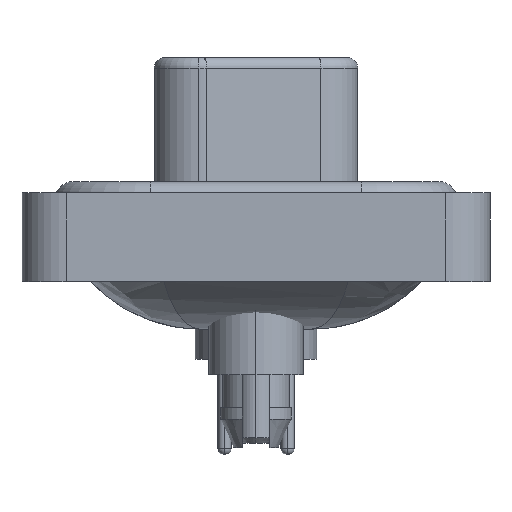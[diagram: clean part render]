
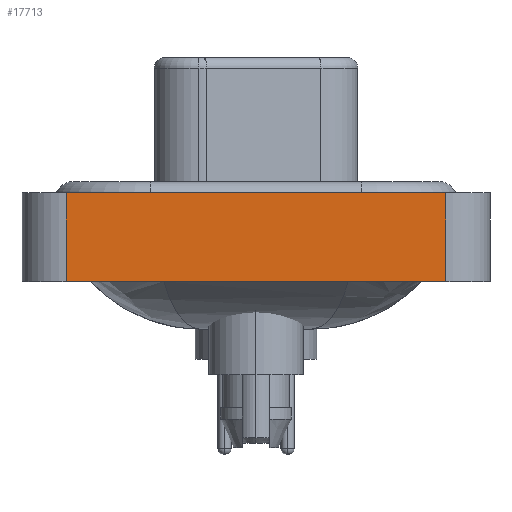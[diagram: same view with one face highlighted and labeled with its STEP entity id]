
A CAD part, left-side view. The second image highlights one B-rep face of the part: STEP entity #17713.
In plain terms, the highlighted planar face has unit normal (-1, 0, 0).
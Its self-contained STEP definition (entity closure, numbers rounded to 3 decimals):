
#1479 = VECTOR ( 'NONE', #15555, 1000. ) ;
#1630 = LINE ( 'NONE', #17493, #13610 ) ;
#1806 = PLANE ( 'NONE',  #7058 ) ;
#2822 = EDGE_LOOP ( 'NONE', ( #3918, #4203, #17969, #15794 ) ) ;
#3918 = ORIENTED_EDGE ( 'NONE', *, *, #9769, .T. ) ;
#4203 = ORIENTED_EDGE ( 'NONE', *, *, #18684, .F. ) ;
#5059 = VERTEX_POINT ( 'NONE', #7297 ) ;
#5425 = CARTESIAN_POINT ( 'NONE',  ( -7.35, -8.55, -3.6 ) ) ;
#6991 = CARTESIAN_POINT ( 'NONE',  ( -7.35, -8.55, -3.6 ) ) ;
#7058 = AXIS2_PLACEMENT_3D ( 'NONE', #6991, #20671, #15852 ) ;
#7297 = CARTESIAN_POINT ( 'NONE',  ( -7.35, -8.55, 0.4 ) ) ;
#8359 = CARTESIAN_POINT ( 'NONE',  ( -7.35, -8.55, -3.6 ) ) ;
#8612 = CARTESIAN_POINT ( 'NONE',  ( -7.35, 8.55, -3.6 ) ) ;
#9769 = EDGE_CURVE ( 'NONE', #21644, #5059, #1630, .T. ) ;
#9813 = EDGE_CURVE ( 'NONE', #21570, #21644, #10720, .T. ) ;
#10720 = LINE ( 'NONE', #5425, #1479 ) ;
#10827 = CARTESIAN_POINT ( 'NONE',  ( -7.35, -8.55, 0.4 ) ) ;
#12209 = CARTESIAN_POINT ( 'NONE',  ( -7.35, 8.55, 0.4 ) ) ;
#13549 = FACE_OUTER_BOUND ( 'NONE', #2822, .T. ) ;
#13610 = VECTOR ( 'NONE', #14170, 1000. ) ;
#14170 = DIRECTION ( 'NONE',  ( 0., 0., 1. ) ) ;
#15555 = DIRECTION ( 'NONE',  ( 0., -1., 0. ) ) ;
#15794 = ORIENTED_EDGE ( 'NONE', *, *, #9813, .T. ) ;
#15852 = DIRECTION ( 'NONE',  ( 0., 0., 1. ) ) ;
#16077 = VERTEX_POINT ( 'NONE', #12209 ) ;
#16282 = VECTOR ( 'NONE', #16551, 1000. ) ;
#16551 = DIRECTION ( 'NONE',  ( 0., -1., 0. ) ) ;
#16575 = VECTOR ( 'NONE', #22518, 1000. ) ;
#17493 = CARTESIAN_POINT ( 'NONE',  ( -7.35, -8.55, -3.6 ) ) ;
#17713 = ADVANCED_FACE ( 'NONE', ( #13549 ), #1806, .T. ) ;
#17969 = ORIENTED_EDGE ( 'NONE', *, *, #18924, .F. ) ;
#18684 = EDGE_CURVE ( 'NONE', #16077, #5059, #19543, .T. ) ;
#18924 = EDGE_CURVE ( 'NONE', #21570, #16077, #20674, .T. ) ;
#19543 = LINE ( 'NONE', #10827, #16282 ) ;
#20671 = DIRECTION ( 'NONE',  ( -1., 0., 0. ) ) ;
#20674 = LINE ( 'NONE', #8612, #16575 ) ;
#21570 = VERTEX_POINT ( 'NONE', #22037 ) ;
#21644 = VERTEX_POINT ( 'NONE', #8359 ) ;
#22037 = CARTESIAN_POINT ( 'NONE',  ( -7.35, 8.55, -3.6 ) ) ;
#22518 = DIRECTION ( 'NONE',  ( 0., 0., 1. ) ) ;
